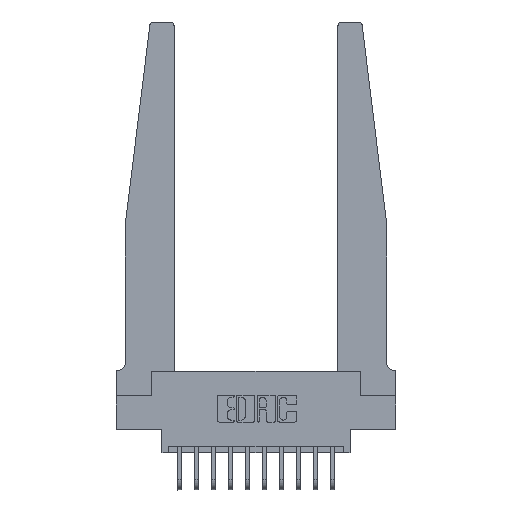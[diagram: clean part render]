
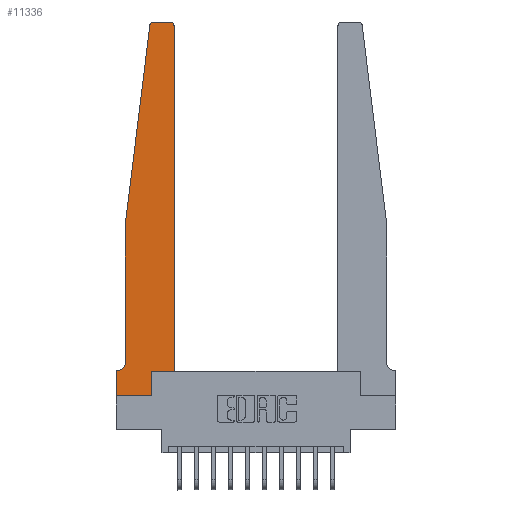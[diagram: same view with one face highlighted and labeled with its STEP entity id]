
A CAD part, top view. The second image highlights one B-rep face of the part: STEP entity #11336.
In plain terms, the highlighted planar face has unit normal (0, 0, 1).
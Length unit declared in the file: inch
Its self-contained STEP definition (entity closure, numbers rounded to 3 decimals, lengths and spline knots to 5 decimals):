
#404 = EDGE_CURVE ( 'NONE', #9157, #13688, #5223, .T. ) ;
#471 = VERTEX_POINT ( 'NONE', #8867 ) ;
#486 = CARTESIAN_POINT ( 'NONE',  ( 0.425, 2.72, 0.37 ) ) ;
#616 = CARTESIAN_POINT ( 'NONE',  ( 0.27653, 2.72, 0.37 ) ) ;
#810 = VERTEX_POINT ( 'NONE', #8615 ) ;
#1138 = VECTOR ( 'NONE', #1725, 39.37008 ) ;
#1470 = CARTESIAN_POINT ( 'NONE',  ( 0.425, 0.18, 0.37 ) ) ;
#1675 = DIRECTION ( 'NONE',  ( 0., -1., 0. ) ) ;
#1705 = ORIENTED_EDGE ( 'NONE', *, *, #404, .T. ) ;
#1725 = DIRECTION ( 'NONE',  ( -1., 0., 0. ) ) ;
#1802 = DIRECTION ( 'NONE',  ( 0., -1., 0. ) ) ;
#1836 = ORIENTED_EDGE ( 'NONE', *, *, #11837, .T. ) ;
#1845 = CARTESIAN_POINT ( 'NONE',  ( 0., 0., 0.37 ) ) ;
#1930 = LINE ( 'NONE', #1845, #6079 ) ;
#2073 = EDGE_CURVE ( 'NONE', #810, #15121, #2394, .T. ) ;
#2124 = AXIS2_PLACEMENT_3D ( 'NONE', #14755, #8640, #2732 ) ;
#2394 = LINE ( 'NONE', #8772, #8258 ) ;
#2400 = AXIS2_PLACEMENT_3D ( 'NONE', #11381, #3721, #11460 ) ;
#2452 = DIRECTION ( 'NONE',  ( 1., 0., 0. ) ) ;
#2732 = DIRECTION ( 'NONE',  ( -1., 0., 0. ) ) ;
#3193 = CIRCLE ( 'NONE', #2400, 0.03 ) ;
#3273 = LINE ( 'NONE', #7247, #5244 ) ;
#3629 = ORIENTED_EDGE ( 'NONE', *, *, #3736, .T. ) ;
#3645 = CARTESIAN_POINT ( 'NONE',  ( 0.425, 0.18, 0.37 ) ) ;
#3721 = DIRECTION ( 'NONE',  ( 0., 0., 1. ) ) ;
#3736 = EDGE_CURVE ( 'NONE', #13006, #10786, #5509, .T. ) ;
#3847 = EDGE_CURVE ( 'NONE', #5103, #12383, #14774, .T. ) ;
#3900 = EDGE_CURVE ( 'NONE', #12383, #9028, #3193, .T. ) ;
#4142 = CARTESIAN_POINT ( 'NONE',  ( 0.425, 0.18, 0.37 ) ) ;
#4190 = EDGE_CURVE ( 'NONE', #10786, #14563, #7030, .T. ) ;
#4302 = CARTESIAN_POINT ( 'NONE',  ( 0.065, 0.1875, 0.37 ) ) ;
#4580 = CARTESIAN_POINT ( 'NONE',  ( 0.065, 0.2375, 0.37 ) ) ;
#4617 = VERTEX_POINT ( 'NONE', #7898 ) ;
#4639 = EDGE_CURVE ( 'NONE', #471, #4617, #5266, .T. ) ;
#4665 = DIRECTION ( 'NONE',  ( 1., 0., 0. ) ) ;
#4887 = ORIENTED_EDGE ( 'NONE', *, *, #3900, .T. ) ;
#5103 = VERTEX_POINT ( 'NONE', #4142 ) ;
#5215 = CARTESIAN_POINT ( 'NONE',  ( 0., 0.1875, 0.37 ) ) ;
#5223 = LINE ( 'NONE', #11357, #9641 ) ;
#5244 = VECTOR ( 'NONE', #15857, 39.37008 ) ;
#5266 = CIRCLE ( 'NONE', #14302, 0.03 ) ;
#5388 = EDGE_LOOP ( 'NONE', ( #1836, #13275, #10716, #3629, #12310, #12723, #1705, #14718, #11222, #5796, #9944, #4887 ) ) ;
#5509 = LINE ( 'NONE', #11872, #9374 ) ;
#5796 = ORIENTED_EDGE ( 'NONE', *, *, #10224, .T. ) ;
#6079 = VECTOR ( 'NONE', #10407, 39.37008 ) ;
#6506 = CARTESIAN_POINT ( 'NONE',  ( 0.2605, 0.18, 0.37 ) ) ;
#6785 = DIRECTION ( 'NONE',  ( -1., 0., 0. ) ) ;
#7030 = CIRCLE ( 'NONE', #2124, 0.05 ) ;
#7247 = CARTESIAN_POINT ( 'NONE',  ( 0.065, 1.25, 0.37 ) ) ;
#7259 = CARTESIAN_POINT ( 'NONE',  ( 0., 0., 0.37 ) ) ;
#7741 = DIRECTION ( 'NONE',  ( 1., 0., 0. ) ) ;
#7898 = CARTESIAN_POINT ( 'NONE',  ( 0.24675, 2.72367, 0.37 ) ) ;
#8225 = PLANE ( 'NONE',  #14045 ) ;
#8258 = VECTOR ( 'NONE', #10946, 39.37008 ) ;
#8609 = EDGE_CURVE ( 'NONE', #14563, #9157, #12946, .T. ) ;
#8615 = CARTESIAN_POINT ( 'NONE',  ( 0.2605, 0., 0.37 ) ) ;
#8640 = DIRECTION ( 'NONE',  ( 0., 0., -1. ) ) ;
#8656 = DIRECTION ( 'NONE',  ( 0., 1., 0. ) ) ;
#8772 = CARTESIAN_POINT ( 'NONE',  ( 0.2605, 0.18, 0.37 ) ) ;
#8867 = CARTESIAN_POINT ( 'NONE',  ( 0.27653, 2.75, 0.37 ) ) ;
#9028 = VERTEX_POINT ( 'NONE', #14589 ) ;
#9157 = VERTEX_POINT ( 'NONE', #5215 ) ;
#9282 = LINE ( 'NONE', #15314, #13267 ) ;
#9374 = VECTOR ( 'NONE', #1802, 39.37008 ) ;
#9641 = VECTOR ( 'NONE', #1675, 39.37008 ) ;
#9881 = CARTESIAN_POINT ( 'NONE',  ( 0.015, 0.1875, 0.37 ) ) ;
#9883 = VECTOR ( 'NONE', #2452, 39.37008 ) ;
#9944 = ORIENTED_EDGE ( 'NONE', *, *, #3847, .T. ) ;
#10224 = EDGE_CURVE ( 'NONE', #15121, #5103, #12607, .T. ) ;
#10407 = DIRECTION ( 'NONE',  ( 1., 0., 0. ) ) ;
#10716 = ORIENTED_EDGE ( 'NONE', *, *, #10750, .T. ) ;
#10750 = EDGE_CURVE ( 'NONE', #4617, #13006, #3273, .T. ) ;
#10786 = VERTEX_POINT ( 'NONE', #4580 ) ;
#10946 = DIRECTION ( 'NONE',  ( 0., 1., 0. ) ) ;
#11222 = ORIENTED_EDGE ( 'NONE', *, *, #2073, .T. ) ;
#11336 = ADVANCED_FACE ( 'NONE', ( #14273 ), #8225, .T. ) ;
#11357 = CARTESIAN_POINT ( 'NONE',  ( 0., 0., 0.37 ) ) ;
#11381 = CARTESIAN_POINT ( 'NONE',  ( 0.395, 2.72, 0.37 ) ) ;
#11460 = DIRECTION ( 'NONE',  ( 1., 0., 0. ) ) ;
#11837 = EDGE_CURVE ( 'NONE', #9028, #471, #9282, .T. ) ;
#11872 = CARTESIAN_POINT ( 'NONE',  ( 0.065, 1.25, 0.37 ) ) ;
#12288 = EDGE_CURVE ( 'NONE', #13688, #810, #1930, .T. ) ;
#12310 = ORIENTED_EDGE ( 'NONE', *, *, #4190, .T. ) ;
#12383 = VERTEX_POINT ( 'NONE', #486 ) ;
#12607 = LINE ( 'NONE', #3645, #9883 ) ;
#12723 = ORIENTED_EDGE ( 'NONE', *, *, #8609, .T. ) ;
#12752 = VECTOR ( 'NONE', #8656, 39.37008 ) ;
#12871 = CARTESIAN_POINT ( 'NONE',  ( 0.065, 1.25, 0.37 ) ) ;
#12946 = LINE ( 'NONE', #4302, #1138 ) ;
#13006 = VERTEX_POINT ( 'NONE', #12871 ) ;
#13267 = VECTOR ( 'NONE', #6785, 39.37008 ) ;
#13275 = ORIENTED_EDGE ( 'NONE', *, *, #4639, .T. ) ;
#13688 = VERTEX_POINT ( 'NONE', #7259 ) ;
#14045 = AXIS2_PLACEMENT_3D ( 'NONE', #14509, #15605, #4665 ) ;
#14273 = FACE_OUTER_BOUND ( 'NONE', #5388, .T. ) ;
#14302 = AXIS2_PLACEMENT_3D ( 'NONE', #616, #15355, #7741 ) ;
#14509 = CARTESIAN_POINT ( 'NONE',  ( 0., 0.1875, 0.37 ) ) ;
#14563 = VERTEX_POINT ( 'NONE', #9881 ) ;
#14589 = CARTESIAN_POINT ( 'NONE',  ( 0.395, 2.75, 0.37 ) ) ;
#14718 = ORIENTED_EDGE ( 'NONE', *, *, #12288, .T. ) ;
#14755 = CARTESIAN_POINT ( 'NONE',  ( 0.015, 0.2375, 0.37 ) ) ;
#14774 = LINE ( 'NONE', #1470, #12752 ) ;
#15121 = VERTEX_POINT ( 'NONE', #6506 ) ;
#15314 = CARTESIAN_POINT ( 'NONE',  ( 0.25, 2.75, 0.37 ) ) ;
#15355 = DIRECTION ( 'NONE',  ( 0., 0., 1. ) ) ;
#15605 = DIRECTION ( 'NONE',  ( 0., 0., 1. ) ) ;
#15857 = DIRECTION ( 'NONE',  ( -0.122, -0.992, 0. ) ) ;
